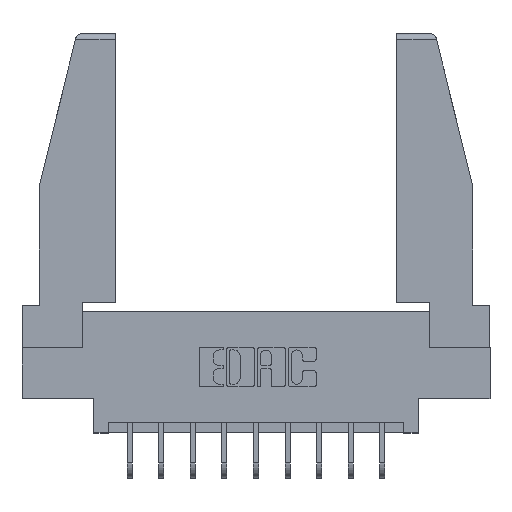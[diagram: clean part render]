
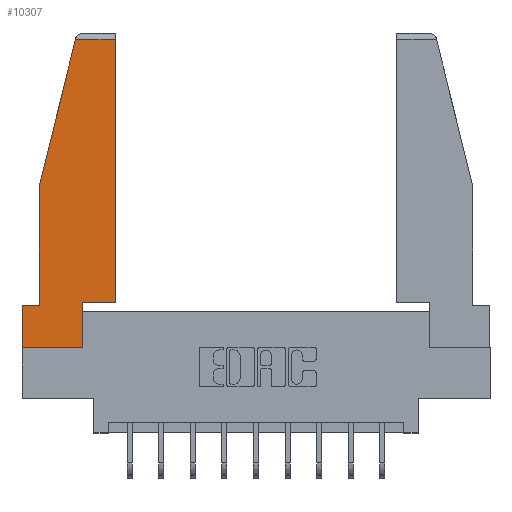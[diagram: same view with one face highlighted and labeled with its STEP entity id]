
A CAD part, top view. The second image highlights one B-rep face of the part: STEP entity #10307.
In plain terms, the highlighted planar face has unit normal (0, 0, 1).
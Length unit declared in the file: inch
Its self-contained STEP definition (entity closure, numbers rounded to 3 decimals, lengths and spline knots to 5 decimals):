
#476 = ORIENTED_EDGE ( 'NONE', *, *, #9297, .T. ) ;
#598 = CARTESIAN_POINT ( 'NONE',  ( 0.2636, 1.52, 0. ) ) ;
#832 = ORIENTED_EDGE ( 'NONE', *, *, #11155, .T. ) ;
#881 = AXIS2_PLACEMENT_3D ( 'NONE', #1936, #15191, #11775 ) ;
#1010 = ORIENTED_EDGE ( 'NONE', *, *, #12757, .T. ) ;
#1028 = LINE ( 'NONE', #12860, #5940 ) ;
#1055 = VERTEX_POINT ( 'NONE', #2290 ) ;
#1198 = DIRECTION ( 'NONE',  ( 0., 1., 0. ) ) ;
#1290 = VECTOR ( 'NONE', #8911, 39.37008 ) ;
#1598 = VERTEX_POINT ( 'NONE', #14299 ) ;
#1634 = LINE ( 'NONE', #4834, #14112 ) ;
#1936 = CARTESIAN_POINT ( 'NONE',  ( 0., 0., 0. ) ) ;
#2072 = ORIENTED_EDGE ( 'NONE', *, *, #2137, .T. ) ;
#2137 = EDGE_CURVE ( 'NONE', #11230, #1055, #4062, .T. ) ;
#2192 = VECTOR ( 'NONE', #13315, 39.37008 ) ;
#2290 = CARTESIAN_POINT ( 'NONE',  ( 0.086, 0.8, 0. ) ) ;
#2442 = VECTOR ( 'NONE', #3124, 39.37008 ) ;
#2650 = CARTESIAN_POINT ( 'NONE',  ( 0.271, 1.55, 0. ) ) ;
#2751 = CARTESIAN_POINT ( 'NONE',  ( 0., 0.21, 0. ) ) ;
#2932 = FACE_OUTER_BOUND ( 'NONE', #12137, .T. ) ;
#3124 = DIRECTION ( 'NONE',  ( -1., 0., 0. ) ) ;
#3252 = LINE ( 'NONE', #5510, #13818 ) ;
#3684 = VECTOR ( 'NONE', #13437, 39.37008 ) ;
#3988 = VERTEX_POINT ( 'NONE', #14177 ) ;
#4062 = LINE ( 'NONE', #2650, #3684 ) ;
#4071 = LINE ( 'NONE', #2751, #2192 ) ;
#4168 = EDGE_CURVE ( 'NONE', #3988, #1598, #11391, .T. ) ;
#4736 = DIRECTION ( 'NONE',  ( 0., -1., 0. ) ) ;
#4834 = CARTESIAN_POINT ( 'NONE',  ( 0.297, 0., 0. ) ) ;
#4894 = DIRECTION ( 'NONE',  ( 0., -1., 0. ) ) ;
#4979 = ORIENTED_EDGE ( 'NONE', *, *, #14621, .T. ) ;
#5510 = CARTESIAN_POINT ( 'NONE',  ( 0., 0., 0. ) ) ;
#5624 = PLANE ( 'NONE',  #881 ) ;
#5940 = VECTOR ( 'NONE', #11653, 39.37008 ) ;
#6265 = CARTESIAN_POINT ( 'NONE',  ( 0.086, 0.8, 0. ) ) ;
#6394 = CARTESIAN_POINT ( 'NONE',  ( 0.297, 0., 0. ) ) ;
#6725 = VERTEX_POINT ( 'NONE', #9403 ) ;
#6844 = ORIENTED_EDGE ( 'NONE', *, *, #7914, .T. ) ;
#6942 = VERTEX_POINT ( 'NONE', #8704 ) ;
#6999 = VERTEX_POINT ( 'NONE', #10081 ) ;
#7446 = VERTEX_POINT ( 'NONE', #9850 ) ;
#7883 = CARTESIAN_POINT ( 'NONE',  ( 0., 1.52, 0. ) ) ;
#7914 = EDGE_CURVE ( 'NONE', #9905, #6942, #1634, .T. ) ;
#8182 = VECTOR ( 'NONE', #4736, 39.37008 ) ;
#8422 = EDGE_CURVE ( 'NONE', #6725, #11230, #15294, .T. ) ;
#8704 = CARTESIAN_POINT ( 'NONE',  ( 0.297, 0.223, 0. ) ) ;
#8778 = ORIENTED_EDGE ( 'NONE', *, *, #4168, .T. ) ;
#8911 = DIRECTION ( 'NONE',  ( 0., 1., 0. ) ) ;
#9297 = EDGE_CURVE ( 'NONE', #7446, #6725, #12463, .T. ) ;
#9403 = CARTESIAN_POINT ( 'NONE',  ( 0.461, 1.52, 0. ) ) ;
#9518 = CARTESIAN_POINT ( 'NONE',  ( 0., 0.21, 0. ) ) ;
#9850 = CARTESIAN_POINT ( 'NONE',  ( 0.461, 0.223, 0. ) ) ;
#9905 = VERTEX_POINT ( 'NONE', #6394 ) ;
#10081 = CARTESIAN_POINT ( 'NONE',  ( 0.086, 0.21, 0. ) ) ;
#10307 = ADVANCED_FACE ( 'NONE', ( #2932 ), #5624, .T. ) ;
#10431 = ORIENTED_EDGE ( 'NONE', *, *, #8422, .T. ) ;
#10625 = ORIENTED_EDGE ( 'NONE', *, *, #13912, .T. ) ;
#11155 = EDGE_CURVE ( 'NONE', #6942, #7446, #1028, .T. ) ;
#11230 = VERTEX_POINT ( 'NONE', #598 ) ;
#11391 = LINE ( 'NONE', #9518, #8182 ) ;
#11653 = DIRECTION ( 'NONE',  ( 1., 0., 0. ) ) ;
#11775 = DIRECTION ( 'NONE',  ( 1., 0., 0. ) ) ;
#12137 = EDGE_LOOP ( 'NONE', ( #476, #10431, #2072, #10625, #4979, #8778, #1010, #6844, #832 ) ) ;
#12463 = LINE ( 'NONE', #13588, #1290 ) ;
#12757 = EDGE_CURVE ( 'NONE', #1598, #9905, #3252, .T. ) ;
#12860 = CARTESIAN_POINT ( 'NONE',  ( 0.297, 0.223, 0. ) ) ;
#13315 = DIRECTION ( 'NONE',  ( -1., 0., 0. ) ) ;
#13417 = VECTOR ( 'NONE', #4894, 39.37008 ) ;
#13437 = DIRECTION ( 'NONE',  ( -0.239, -0.971, 0. ) ) ;
#13588 = CARTESIAN_POINT ( 'NONE',  ( 0.461, 0.223, 0. ) ) ;
#13818 = VECTOR ( 'NONE', #13954, 39.37008 ) ;
#13912 = EDGE_CURVE ( 'NONE', #1055, #6999, #15491, .T. ) ;
#13954 = DIRECTION ( 'NONE',  ( 1., 0., 0. ) ) ;
#14112 = VECTOR ( 'NONE', #1198, 39.37008 ) ;
#14177 = CARTESIAN_POINT ( 'NONE',  ( 0., 0.21, 0. ) ) ;
#14299 = CARTESIAN_POINT ( 'NONE',  ( 0., 0., 0. ) ) ;
#14621 = EDGE_CURVE ( 'NONE', #6999, #3988, #4071, .T. ) ;
#15191 = DIRECTION ( 'NONE',  ( 0., 0., 1. ) ) ;
#15294 = LINE ( 'NONE', #7883, #2442 ) ;
#15491 = LINE ( 'NONE', #6265, #13417 ) ;
